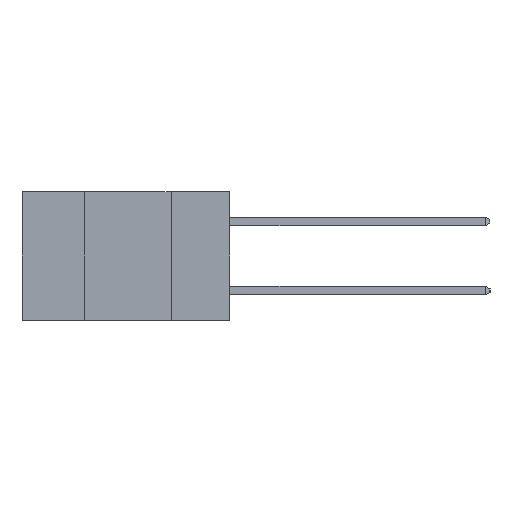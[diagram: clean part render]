
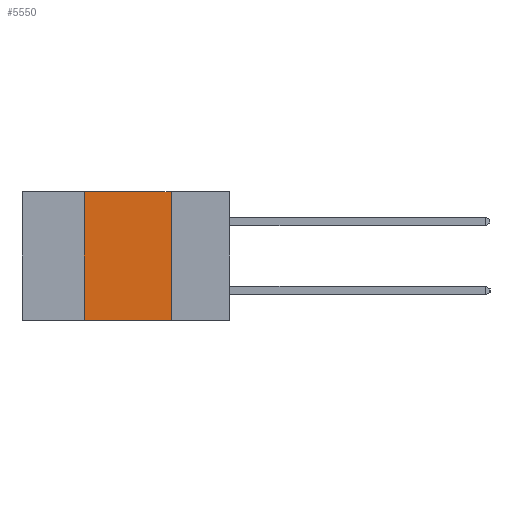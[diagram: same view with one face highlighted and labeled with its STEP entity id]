
A CAD part, left-side view. The second image highlights one B-rep face of the part: STEP entity #5550.
In plain terms, the highlighted planar face has unit normal (-1, 0, 0).
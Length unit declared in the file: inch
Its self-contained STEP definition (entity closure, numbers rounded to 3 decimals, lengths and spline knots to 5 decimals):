
#1227 = CARTESIAN_POINT ( 'NONE',  ( 0., 0.42, -0.37 ) ) ;
#1230 = EDGE_CURVE ( 'NONE', #8079, #2811, #7428, .T. ) ;
#1606 = EDGE_CURVE ( 'NONE', #4863, #2190, #3982, .T. ) ;
#1646 = CARTESIAN_POINT ( 'NONE',  ( 0., 0.6, 0. ) ) ;
#2190 = VERTEX_POINT ( 'NONE', #7444 ) ;
#2356 = CARTESIAN_POINT ( 'NONE',  ( 0., 0.6, 0. ) ) ;
#2406 = ORIENTED_EDGE ( 'NONE', *, *, #1606, .T. ) ;
#2428 = CARTESIAN_POINT ( 'NONE',  ( 0., 0.42, -0.37 ) ) ;
#2504 = PLANE ( 'NONE',  #3581 ) ;
#2546 = DIRECTION ( 'NONE',  ( 0., 0., -1. ) ) ;
#2549 = DIRECTION ( 'NONE',  ( 1., 0., 0. ) ) ;
#2811 = VERTEX_POINT ( 'NONE', #5114 ) ;
#2945 = DIRECTION ( 'NONE',  ( 0., -1., 0. ) ) ;
#3425 = LINE ( 'NONE', #6750, #7994 ) ;
#3451 = EDGE_CURVE ( 'NONE', #4863, #8079, #5423, .T. ) ;
#3581 = AXIS2_PLACEMENT_3D ( 'NONE', #1646, #2549, #2546 ) ;
#3598 = VECTOR ( 'NONE', #3958, 39.37008 ) ;
#3958 = DIRECTION ( 'NONE',  ( 0., 0., 1. ) ) ;
#3982 = LINE ( 'NONE', #6518, #7153 ) ;
#4138 = ORIENTED_EDGE ( 'NONE', *, *, #7457, .F. ) ;
#4863 = VERTEX_POINT ( 'NONE', #2428 ) ;
#5114 = CARTESIAN_POINT ( 'NONE',  ( 0., 0.17, 0. ) ) ;
#5361 = FACE_OUTER_BOUND ( 'NONE', #7783, .T. ) ;
#5423 = LINE ( 'NONE', #1227, #3598 ) ;
#5550 = ADVANCED_FACE ( 'NONE', ( #5361 ), #2504, .F. ) ;
#5916 = VECTOR ( 'NONE', #2945, 39.37008 ) ;
#6511 = DIRECTION ( 'NONE',  ( 0., -1., 0. ) ) ;
#6518 = CARTESIAN_POINT ( 'NONE',  ( 0., 0.6, -0.37 ) ) ;
#6745 = ORIENTED_EDGE ( 'NONE', *, *, #1230, .F. ) ;
#6750 = CARTESIAN_POINT ( 'NONE',  ( 0., 0.17, -0.37 ) ) ;
#7153 = VECTOR ( 'NONE', #6511, 39.37008 ) ;
#7428 = LINE ( 'NONE', #2356, #5916 ) ;
#7444 = CARTESIAN_POINT ( 'NONE',  ( 0., 0.17, -0.37 ) ) ;
#7457 = EDGE_CURVE ( 'NONE', #2811, #2190, #3425, .T. ) ;
#7710 = ORIENTED_EDGE ( 'NONE', *, *, #3451, .F. ) ;
#7783 = EDGE_LOOP ( 'NONE', ( #4138, #6745, #7710, #2406 ) ) ;
#7994 = VECTOR ( 'NONE', #8421, 39.37008 ) ;
#8079 = VERTEX_POINT ( 'NONE', #8280 ) ;
#8280 = CARTESIAN_POINT ( 'NONE',  ( 0., 0.42, 0. ) ) ;
#8421 = DIRECTION ( 'NONE',  ( 0., 0., -1. ) ) ;
